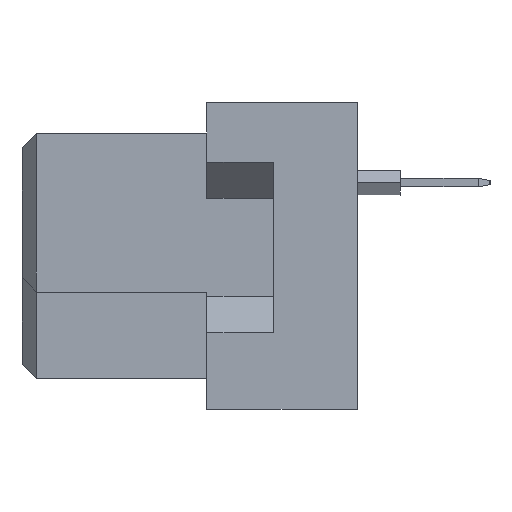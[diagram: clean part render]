
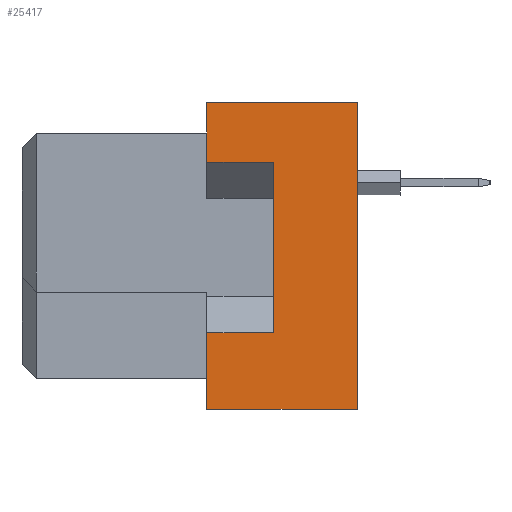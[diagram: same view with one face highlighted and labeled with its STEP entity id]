
A CAD part, left-side view. The second image highlights one B-rep face of the part: STEP entity #25417.
In plain terms, the highlighted planar face has unit normal (-1, 0, 0).
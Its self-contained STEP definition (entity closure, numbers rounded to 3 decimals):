
#1295 = EDGE_CURVE ( 'NONE', #34976, #35585, #6151, .T. ) ;
#2195 = EDGE_CURVE ( 'NONE', #17898, #36807, #35801, .T. ) ;
#2655 = CARTESIAN_POINT ( 'NONE',  ( -47.5, -6.4, -5.3 ) ) ;
#3169 = ORIENTED_EDGE ( 'NONE', *, *, #13313, .F. ) ;
#3751 = DIRECTION ( 'NONE',  ( 0., 0., 1. ) ) ;
#3888 = FACE_OUTER_BOUND ( 'NONE', #17683, .T. ) ;
#4330 = VECTOR ( 'NONE', #12179, 1000. ) ;
#5081 = VECTOR ( 'NONE', #21173, 1000. ) ;
#5265 = LINE ( 'NONE', #37521, #29382 ) ;
#5786 = CARTESIAN_POINT ( 'NONE',  ( -47.5, -8.7, 3.25 ) ) ;
#6151 = LINE ( 'NONE', #17830, #4330 ) ;
#7230 = ORIENTED_EDGE ( 'NONE', *, *, #36271, .F. ) ;
#7539 = CARTESIAN_POINT ( 'NONE',  ( -47.5, -6.4, 3.25 ) ) ;
#8370 = ORIENTED_EDGE ( 'NONE', *, *, #36881, .T. ) ;
#8512 = ORIENTED_EDGE ( 'NONE', *, *, #19549, .F. ) ;
#9172 = DIRECTION ( 'NONE',  ( 0., 0., 1. ) ) ;
#9779 = VERTEX_POINT ( 'NONE', #7539 ) ;
#9899 = DIRECTION ( 'NONE',  ( -1., 0., 0. ) ) ;
#10668 = CARTESIAN_POINT ( 'NONE',  ( -47.5, -6.4, -2.65 ) ) ;
#10901 = DIRECTION ( 'NONE',  ( 0., 1., 0. ) ) ;
#11806 = DIRECTION ( 'NONE',  ( 0., 1., 0. ) ) ;
#11915 = ORIENTED_EDGE ( 'NONE', *, *, #2195, .F. ) ;
#11958 = VERTEX_POINT ( 'NONE', #21248 ) ;
#12030 = ORIENTED_EDGE ( 'NONE', *, *, #28793, .T. ) ;
#12179 = DIRECTION ( 'NONE',  ( 0., 0., 1. ) ) ;
#13313 = EDGE_CURVE ( 'NONE', #9779, #11958, #28210, .T. ) ;
#13804 = VERTEX_POINT ( 'NONE', #37292 ) ;
#14738 = LINE ( 'NONE', #35155, #22459 ) ;
#15117 = VERTEX_POINT ( 'NONE', #32634 ) ;
#15197 = CARTESIAN_POINT ( 'NONE',  ( -47.5, -8.7, -2.65 ) ) ;
#15939 = DIRECTION ( 'NONE',  ( 0., 0., 1. ) ) ;
#16367 = CARTESIAN_POINT ( 'NONE',  ( -47.5, -6.4, -5.3 ) ) ;
#16675 = ORIENTED_EDGE ( 'NONE', *, *, #30429, .T. ) ;
#17683 = EDGE_LOOP ( 'NONE', ( #12030, #31625, #8512, #8370, #16675, #3169, #7230, #11915 ) ) ;
#17830 = CARTESIAN_POINT ( 'NONE',  ( -47.5, -6.4, -5.3 ) ) ;
#17898 = VERTEX_POINT ( 'NONE', #34639 ) ;
#18854 = CARTESIAN_POINT ( 'NONE',  ( -47.5, -11.6, 5.3 ) ) ;
#19549 = EDGE_CURVE ( 'NONE', #15117, #34976, #5265, .T. ) ;
#21173 = DIRECTION ( 'NONE',  ( 0., 1., 0. ) ) ;
#21248 = CARTESIAN_POINT ( 'NONE',  ( -47.5, -6.4, 5.3 ) ) ;
#21534 = LINE ( 'NONE', #24053, #25668 ) ;
#22459 = VECTOR ( 'NONE', #11806, 1000. ) ;
#24053 = CARTESIAN_POINT ( 'NONE',  ( -47.5, -11.6, 5.3 ) ) ;
#25417 = ADVANCED_FACE ( 'NONE', ( #3888 ), #33596, .T. ) ;
#25668 = VECTOR ( 'NONE', #26969, 1000. ) ;
#25862 = DIRECTION ( 'NONE',  ( 0., 1., 0. ) ) ;
#25870 = CARTESIAN_POINT ( 'NONE',  ( -47.5, -8.7, 3.25 ) ) ;
#26969 = DIRECTION ( 'NONE',  ( 0., 0., 1. ) ) ;
#28067 = AXIS2_PLACEMENT_3D ( 'NONE', #18854, #9899, #15939 ) ;
#28210 = LINE ( 'NONE', #16367, #30785 ) ;
#28572 = LINE ( 'NONE', #25870, #30092 ) ;
#28793 = EDGE_CURVE ( 'NONE', #17898, #35585, #35188, .T. ) ;
#28949 = VECTOR ( 'NONE', #9172, 1000. ) ;
#29382 = VECTOR ( 'NONE', #25862, 1000. ) ;
#30092 = VECTOR ( 'NONE', #10901, 1000. ) ;
#30429 = EDGE_CURVE ( 'NONE', #13804, #11958, #14738, .T. ) ;
#30785 = VECTOR ( 'NONE', #3751, 1000. ) ;
#31625 = ORIENTED_EDGE ( 'NONE', *, *, #1295, .F. ) ;
#32634 = CARTESIAN_POINT ( 'NONE',  ( -47.5, -11.6, -5.3 ) ) ;
#33596 = PLANE ( 'NONE',  #28067 ) ;
#34639 = CARTESIAN_POINT ( 'NONE',  ( -47.5, -8.7, -2.65 ) ) ;
#34976 = VERTEX_POINT ( 'NONE', #2655 ) ;
#35155 = CARTESIAN_POINT ( 'NONE',  ( -47.5, -11.6, 5.3 ) ) ;
#35188 = LINE ( 'NONE', #38295, #5081 ) ;
#35585 = VERTEX_POINT ( 'NONE', #10668 ) ;
#35801 = LINE ( 'NONE', #15197, #28949 ) ;
#36271 = EDGE_CURVE ( 'NONE', #36807, #9779, #28572, .T. ) ;
#36807 = VERTEX_POINT ( 'NONE', #5786 ) ;
#36881 = EDGE_CURVE ( 'NONE', #15117, #13804, #21534, .T. ) ;
#37292 = CARTESIAN_POINT ( 'NONE',  ( -47.5, -11.6, 5.3 ) ) ;
#37521 = CARTESIAN_POINT ( 'NONE',  ( -47.5, -11.6, -5.3 ) ) ;
#38295 = CARTESIAN_POINT ( 'NONE',  ( -47.5, -8.7, -2.65 ) ) ;
